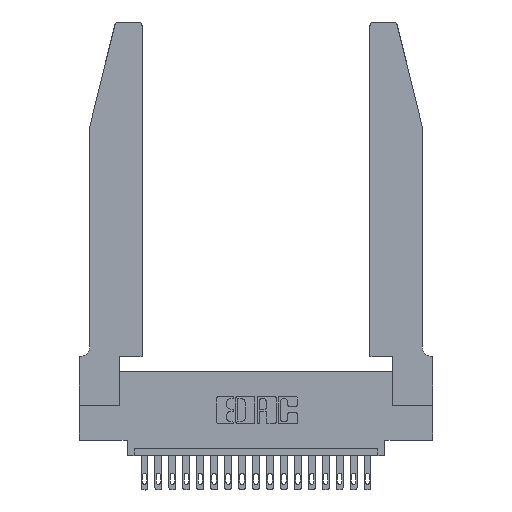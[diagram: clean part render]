
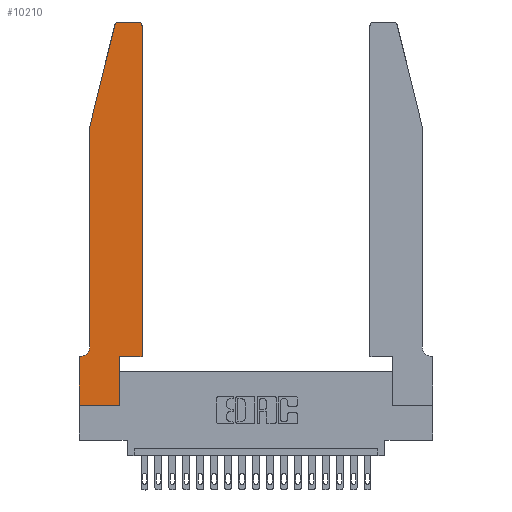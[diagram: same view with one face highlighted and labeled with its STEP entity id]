
A CAD part, top view. The second image highlights one B-rep face of the part: STEP entity #10210.
In plain terms, the highlighted planar face has unit normal (0, 0, 1).
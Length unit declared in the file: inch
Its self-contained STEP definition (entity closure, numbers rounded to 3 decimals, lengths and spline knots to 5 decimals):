
#32 = ORIENTED_EDGE ( 'NONE', *, *, #12196, .T. ) ;
#202 = CARTESIAN_POINT ( 'NONE',  ( 0.4505, 0.35, 0.37 ) ) ;
#238 = ORIENTED_EDGE ( 'NONE', *, *, #6477, .T. ) ;
#471 = VERTEX_POINT ( 'NONE', #12802 ) ;
#620 = VECTOR ( 'NONE', #12522, 39.37008 ) ;
#661 = CARTESIAN_POINT ( 'NONE',  ( 0.0755, 0.42, 0.37 ) ) ;
#824 = CARTESIAN_POINT ( 'NONE',  ( 0., 0.35, 0.37 ) ) ;
#1035 = DIRECTION ( 'NONE',  ( 1., 0., 0. ) ) ;
#1309 = EDGE_CURVE ( 'NONE', #5228, #20626, #7972, .T. ) ;
#1376 = CARTESIAN_POINT ( 'NONE',  ( 0.4505, 2.72, 0.37 ) ) ;
#1386 = EDGE_CURVE ( 'NONE', #9734, #12079, #15537, .T. ) ;
#1790 = CARTESIAN_POINT ( 'NONE',  ( 0.284, 2.72, 0.37 ) ) ;
#1930 = DIRECTION ( 'NONE',  ( 1., 0., 0. ) ) ;
#1969 = ORIENTED_EDGE ( 'NONE', *, *, #12587, .T. ) ;
#2164 = LINE ( 'NONE', #8331, #7232 ) ;
#2191 = EDGE_CURVE ( 'NONE', #7596, #471, #13611, .T. ) ;
#2370 = LINE ( 'NONE', #5909, #620 ) ;
#2818 = VECTOR ( 'NONE', #18861, 39.37008 ) ;
#2913 = LINE ( 'NONE', #19602, #18622 ) ;
#3196 = DIRECTION ( 'NONE',  ( 1., 0., 0. ) ) ;
#3513 = EDGE_CURVE ( 'NONE', #15545, #20114, #2164, .T. ) ;
#4103 = FACE_OUTER_BOUND ( 'NONE', #13524, .T. ) ;
#4192 = DIRECTION ( 'NONE',  ( 0., 0., -1. ) ) ;
#4907 = ORIENTED_EDGE ( 'NONE', *, *, #11797, .T. ) ;
#5107 = LINE ( 'NONE', #13910, #13445 ) ;
#5228 = VERTEX_POINT ( 'NONE', #202 ) ;
#5721 = CARTESIAN_POINT ( 'NONE',  ( 0.0055, 0.35, 0.37 ) ) ;
#5817 = EDGE_CURVE ( 'NONE', #12079, #6628, #10674, .T. ) ;
#5851 = LINE ( 'NONE', #12516, #16495 ) ;
#5909 = CARTESIAN_POINT ( 'NONE',  ( 0., 0., 0.37 ) ) ;
#6477 = EDGE_CURVE ( 'NONE', #20626, #15545, #19012, .T. ) ;
#6508 = ORIENTED_EDGE ( 'NONE', *, *, #1309, .T. ) ;
#6628 = VERTEX_POINT ( 'NONE', #19556 ) ;
#7189 = AXIS2_PLACEMENT_3D ( 'NONE', #14521, #7888, #3196 ) ;
#7203 = DIRECTION ( 'NONE',  ( 0., 1., 0. ) ) ;
#7232 = VECTOR ( 'NONE', #17790, 39.37008 ) ;
#7596 = VERTEX_POINT ( 'NONE', #16192 ) ;
#7697 = VERTEX_POINT ( 'NONE', #9616 ) ;
#7888 = DIRECTION ( 'NONE',  ( 0., 0., 1. ) ) ;
#7972 = LINE ( 'NONE', #10597, #8483 ) ;
#8331 = CARTESIAN_POINT ( 'NONE',  ( 0.2605, 2.75, 0.37 ) ) ;
#8363 = DIRECTION ( 'NONE',  ( 1., 0., 0. ) ) ;
#8483 = VECTOR ( 'NONE', #7203, 39.37008 ) ;
#8910 = DIRECTION ( 'NONE',  ( 1., 0., 0. ) ) ;
#9137 = CIRCLE ( 'NONE', #11634, 0.03 ) ;
#9474 = EDGE_CURVE ( 'NONE', #6628, #7596, #2370, .T. ) ;
#9616 = CARTESIAN_POINT ( 'NONE',  ( 0.25487, 2.72718, 0.37 ) ) ;
#9734 = VERTEX_POINT ( 'NONE', #661 ) ;
#9830 = CARTESIAN_POINT ( 'NONE',  ( 0.2865, 0.35, 0.37 ) ) ;
#10051 = CARTESIAN_POINT ( 'NONE',  ( 0.284, 2.75, 0.37 ) ) ;
#10210 = ADVANCED_FACE ( 'NONE', ( #4103 ), #10542, .T. ) ;
#10542 = PLANE ( 'NONE',  #20122 ) ;
#10597 = CARTESIAN_POINT ( 'NONE',  ( 0.4505, 0.35, 0.37 ) ) ;
#10674 = LINE ( 'NONE', #13614, #2818 ) ;
#11107 = EDGE_CURVE ( 'NONE', #13400, #5228, #5851, .T. ) ;
#11628 = DIRECTION ( 'NONE',  ( 0., 0., 1. ) ) ;
#11634 = AXIS2_PLACEMENT_3D ( 'NONE', #1790, #11628, #1930 ) ;
#11797 = EDGE_CURVE ( 'NONE', #471, #13400, #5107, .T. ) ;
#12079 = VERTEX_POINT ( 'NONE', #5721 ) ;
#12196 = EDGE_CURVE ( 'NONE', #20114, #7697, #9137, .T. ) ;
#12343 = ORIENTED_EDGE ( 'NONE', *, *, #9474, .T. ) ;
#12370 = ORIENTED_EDGE ( 'NONE', *, *, #18177, .T. ) ;
#12516 = CARTESIAN_POINT ( 'NONE',  ( 0.4505, 0.35, 0.37 ) ) ;
#12522 = DIRECTION ( 'NONE',  ( 0., -1., 0. ) ) ;
#12587 = EDGE_CURVE ( 'NONE', #15928, #9734, #20538, .T. ) ;
#12802 = CARTESIAN_POINT ( 'NONE',  ( 0.2865, 0., 0.37 ) ) ;
#13163 = VECTOR ( 'NONE', #16341, 39.37008 ) ;
#13353 = ORIENTED_EDGE ( 'NONE', *, *, #2191, .T. ) ;
#13400 = VERTEX_POINT ( 'NONE', #9830 ) ;
#13445 = VECTOR ( 'NONE', #20595, 39.37008 ) ;
#13470 = CARTESIAN_POINT ( 'NONE',  ( 0.4205, 2.75, 0.37 ) ) ;
#13524 = EDGE_LOOP ( 'NONE', ( #15135, #32, #12370, #1969, #18623, #20299, #12343, #13353, #4907, #14980, #6508, #238 ) ) ;
#13611 = LINE ( 'NONE', #16414, #17419 ) ;
#13614 = CARTESIAN_POINT ( 'NONE',  ( 0.0755, 0.35, 0.37 ) ) ;
#13910 = CARTESIAN_POINT ( 'NONE',  ( 0.2865, 0.35, 0.37 ) ) ;
#14521 = CARTESIAN_POINT ( 'NONE',  ( 0.4205, 2.72, 0.37 ) ) ;
#14693 = CARTESIAN_POINT ( 'NONE',  ( 0.0755, 2., 0.37 ) ) ;
#14980 = ORIENTED_EDGE ( 'NONE', *, *, #11107, .T. ) ;
#15135 = ORIENTED_EDGE ( 'NONE', *, *, #3513, .T. ) ;
#15530 = DIRECTION ( 'NONE',  ( -1., 0., 0. ) ) ;
#15537 = CIRCLE ( 'NONE', #15803, 0.07 ) ;
#15545 = VERTEX_POINT ( 'NONE', #13470 ) ;
#15803 = AXIS2_PLACEMENT_3D ( 'NONE', #20655, #4192, #15530 ) ;
#15928 = VERTEX_POINT ( 'NONE', #16015 ) ;
#16015 = CARTESIAN_POINT ( 'NONE',  ( 0.0755, 2., 0.37 ) ) ;
#16192 = CARTESIAN_POINT ( 'NONE',  ( 0., 0., 0.37 ) ) ;
#16341 = DIRECTION ( 'NONE',  ( 0., -1., 0. ) ) ;
#16414 = CARTESIAN_POINT ( 'NONE',  ( 0., 0., 0.37 ) ) ;
#16495 = VECTOR ( 'NONE', #1035, 39.37008 ) ;
#17419 = VECTOR ( 'NONE', #8363, 39.37008 ) ;
#17790 = DIRECTION ( 'NONE',  ( -1., 0., 0. ) ) ;
#18177 = EDGE_CURVE ( 'NONE', #7697, #15928, #2913, .T. ) ;
#18379 = DIRECTION ( 'NONE',  ( -0.239, -0.971, 0. ) ) ;
#18600 = DIRECTION ( 'NONE',  ( 0., 0., 1. ) ) ;
#18622 = VECTOR ( 'NONE', #18379, 39.37008 ) ;
#18623 = ORIENTED_EDGE ( 'NONE', *, *, #1386, .T. ) ;
#18861 = DIRECTION ( 'NONE',  ( -1., 0., 0. ) ) ;
#19012 = CIRCLE ( 'NONE', #7189, 0.03 ) ;
#19556 = CARTESIAN_POINT ( 'NONE',  ( 0., 0.35, 0.37 ) ) ;
#19602 = CARTESIAN_POINT ( 'NONE',  ( 0.0755, 2., 0.37 ) ) ;
#20114 = VERTEX_POINT ( 'NONE', #10051 ) ;
#20122 = AXIS2_PLACEMENT_3D ( 'NONE', #824, #18600, #8910 ) ;
#20299 = ORIENTED_EDGE ( 'NONE', *, *, #5817, .T. ) ;
#20538 = LINE ( 'NONE', #14693, #13163 ) ;
#20595 = DIRECTION ( 'NONE',  ( 0., 1., 0. ) ) ;
#20626 = VERTEX_POINT ( 'NONE', #1376 ) ;
#20655 = CARTESIAN_POINT ( 'NONE',  ( 0.0055, 0.42, 0.37 ) ) ;
